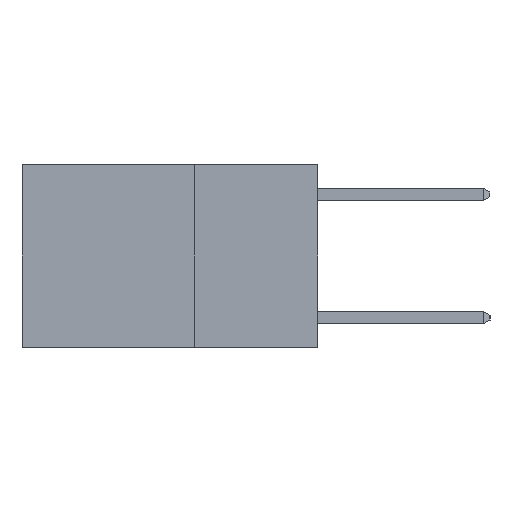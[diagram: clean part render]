
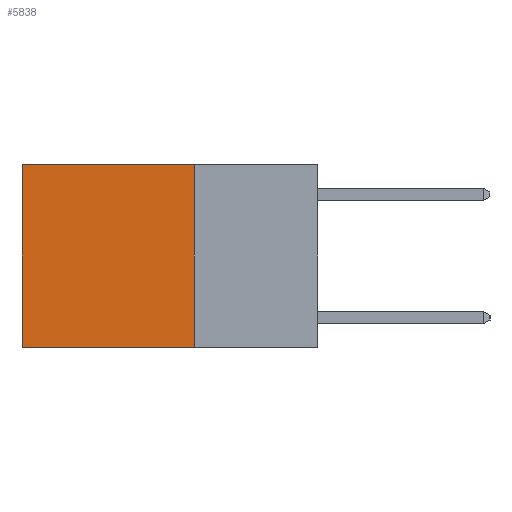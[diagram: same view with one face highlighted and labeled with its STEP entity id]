
A CAD part, left-side view. The second image highlights one B-rep face of the part: STEP entity #5838.
In plain terms, the highlighted planar face has unit normal (-1, 0, 0).
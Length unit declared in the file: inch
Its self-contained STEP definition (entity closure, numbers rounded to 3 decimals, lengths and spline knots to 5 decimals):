
#357 = EDGE_LOOP ( 'NONE', ( #8090, #8590, #5966, #613 ) ) ;
#613 = ORIENTED_EDGE ( 'NONE', *, *, #2078, .T. ) ;
#920 = DIRECTION ( 'NONE',  ( 0., 0., -1. ) ) ;
#1041 = DIRECTION ( 'NONE',  ( 0., 0., -1. ) ) ;
#1790 = PLANE ( 'NONE',  #7711 ) ;
#2078 = EDGE_CURVE ( 'NONE', #9678, #5503, #9430, .T. ) ;
#2345 = CARTESIAN_POINT ( 'NONE',  ( 0.2625, 0.25, 0. ) ) ;
#2452 = DIRECTION ( 'NONE',  ( 0., 1., 0. ) ) ;
#2678 = DIRECTION ( 'NONE',  ( 0., 0., -1. ) ) ;
#2685 = CARTESIAN_POINT ( 'NONE',  ( 0.2625, 0.6, 0. ) ) ;
#4463 = VERTEX_POINT ( 'NONE', #8133 ) ;
#4498 = EDGE_CURVE ( 'NONE', #9678, #4463, #5284, .T. ) ;
#4561 = VECTOR ( 'NONE', #1041, 39.37008 ) ;
#5104 = EDGE_CURVE ( 'NONE', #4463, #6503, #7732, .T. ) ;
#5284 = LINE ( 'NONE', #5818, #5534 ) ;
#5469 = VECTOR ( 'NONE', #2452, 39.37008 ) ;
#5503 = VERTEX_POINT ( 'NONE', #7061 ) ;
#5534 = VECTOR ( 'NONE', #920, 39.37008 ) ;
#5818 = CARTESIAN_POINT ( 'NONE',  ( 0.2625, 0.25, 0. ) ) ;
#5838 = ADVANCED_FACE ( 'NONE', ( #7097 ), #1790, .F. ) ;
#5895 = VECTOR ( 'NONE', #10549, 39.37008 ) ;
#5897 = CARTESIAN_POINT ( 'NONE',  ( 0.2625, 0.25, 0. ) ) ;
#5966 = ORIENTED_EDGE ( 'NONE', *, *, #4498, .F. ) ;
#6503 = VERTEX_POINT ( 'NONE', #9202 ) ;
#6668 = LINE ( 'NONE', #2685, #4561 ) ;
#7061 = CARTESIAN_POINT ( 'NONE',  ( 0.2625, 0.6, 0. ) ) ;
#7097 = FACE_OUTER_BOUND ( 'NONE', #357, .T. ) ;
#7457 = DIRECTION ( 'NONE',  ( 1., 0., 0. ) ) ;
#7711 = AXIS2_PLACEMENT_3D ( 'NONE', #5897, #7457, #2678 ) ;
#7732 = LINE ( 'NONE', #8088, #5895 ) ;
#8088 = CARTESIAN_POINT ( 'NONE',  ( 0.2625, 0.25, -0.37 ) ) ;
#8090 = ORIENTED_EDGE ( 'NONE', *, *, #8557, .T. ) ;
#8133 = CARTESIAN_POINT ( 'NONE',  ( 0.2625, 0.25, -0.37 ) ) ;
#8557 = EDGE_CURVE ( 'NONE', #5503, #6503, #6668, .T. ) ;
#8590 = ORIENTED_EDGE ( 'NONE', *, *, #5104, .F. ) ;
#9202 = CARTESIAN_POINT ( 'NONE',  ( 0.2625, 0.6, -0.37 ) ) ;
#9266 = CARTESIAN_POINT ( 'NONE',  ( 0.2625, 0.25, 0. ) ) ;
#9430 = LINE ( 'NONE', #2345, #5469 ) ;
#9678 = VERTEX_POINT ( 'NONE', #9266 ) ;
#10549 = DIRECTION ( 'NONE',  ( 0., 1., 0. ) ) ;
